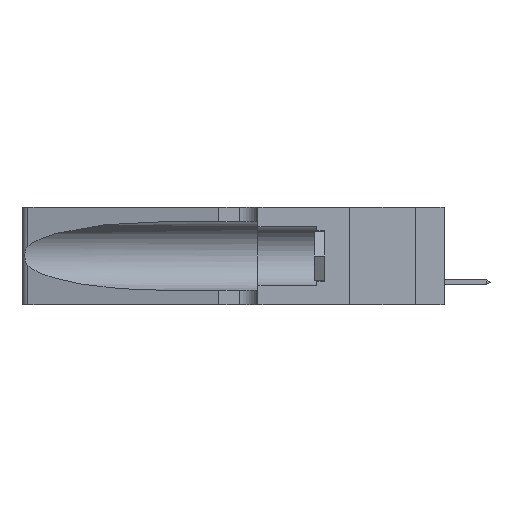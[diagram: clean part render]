
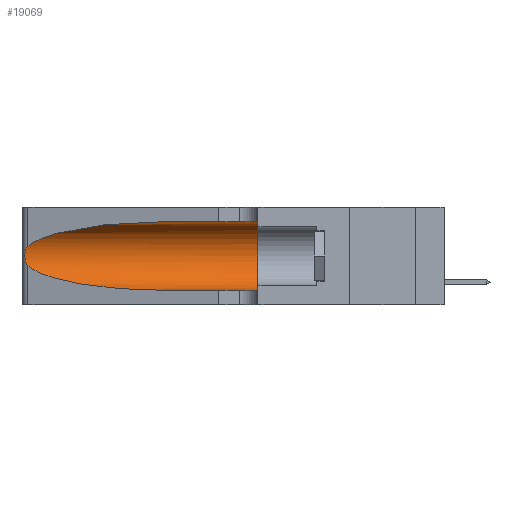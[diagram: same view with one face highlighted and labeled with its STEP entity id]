
A CAD part, left-side view. The second image highlights one B-rep face of the part: STEP entity #19069.
In plain terms, the highlighted cylindrical face has radius 3.308 mm (diameter 6.617 mm), a partial arc.
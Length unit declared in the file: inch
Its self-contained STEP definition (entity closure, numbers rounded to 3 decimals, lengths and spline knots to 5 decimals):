
#57 = CYLINDRICAL_SURFACE ( 'NONE', #22154, 0.13025 ) ;
#59 = CARTESIAN_POINT ( 'NONE',  ( 0.25639, 1.23184, 0.21858 ) ) ;
#171 = CARTESIAN_POINT ( 'NONE',  ( 0.18966, 0.96281, 0.05475 ) ) ;
#181 = CARTESIAN_POINT ( 'NONE',  ( 0.1305, 0.35, 0.31525 ) ) ;
#668 = DIRECTION ( 'NONE',  ( 0., -1., 0. ) ) ;
#1163 = VERTEX_POINT ( 'NONE', #20608 ) ;
#1965 = CARTESIAN_POINT ( 'NONE',  ( 0.1305, 1.61858, 0.05475 ) ) ;
#2052 = CARTESIAN_POINT ( 'NONE',  ( 0.1305, 0.35, 0.05475 ) ) ;
#2307 = CARTESIAN_POINT ( 'NONE',  ( 0.25639, 1.23186, 0.15144 ) ) ;
#3099 = VECTOR ( 'NONE', #668, 39.37008 ) ;
#3864 = EDGE_LOOP ( 'NONE', ( #15923, #24804, #15030, #12598, #13531, #11476 ) ) ;
#4411 = CARTESIAN_POINT ( 'NONE',  ( 0.25487, 1.22718, 0.14631 ) ) ;
#5501 = B_SPLINE_CURVE_WITH_KNOTS ( 'NONE', 3,
 ( #21310, #14853, #59, #8733, #10868, #6243, #8461, #10586, #12723, #23414, #21129, #2307, #16975, #4411 ),
 .UNSPECIFIED., .F., .F.,
 ( 4, 2, 2, 2, 2, 2, 4 ),
 ( 0., 0.00027, 0.00053, 0.00107, 0.0016, 0.00187, 0.00214 ),
 .UNSPECIFIED. ) ;
#6243 = CARTESIAN_POINT ( 'NONE',  ( 0.26018, 1.23835, 0.19895 ) ) ;
#6531 = CARTESIAN_POINT ( 'NONE',  ( 0.1305, 0.72297, 0.05475 ) ) ;
#7125 = CARTESIAN_POINT ( 'NONE',  ( 0.25487, 1.22718, 0.14631 ) ) ;
#7676 = FACE_OUTER_BOUND ( 'NONE', #3864, .T. ) ;
#7796 = CARTESIAN_POINT ( 'NONE',  ( 0.18966, 0.96281, 0.31525 ) ) ;
#8120 = DIRECTION ( 'NONE',  ( 0., -1., 0. ) ) ;
#8461 = CARTESIAN_POINT ( 'NONE',  ( 0.26075, 1.23896, 0.19203 ) ) ;
#8733 = CARTESIAN_POINT ( 'NONE',  ( 0.25787, 1.23484, 0.2124 ) ) ;
#10179 = DIRECTION ( 'NONE',  ( 0., 1., 0. ) ) ;
#10402 = CARTESIAN_POINT ( 'NONE',  ( 0.1305, 1.61858, 0.185 ) ) ;
#10586 = CARTESIAN_POINT ( 'NONE',  ( 0.26075, 1.23896, 0.178 ) ) ;
#10868 = CARTESIAN_POINT ( 'NONE',  ( 0.25854, 1.2359, 0.20912 ) ) ;
#11476 = ORIENTED_EDGE ( 'NONE', *, *, #18716, .F. ) ;
#12152 = CARTESIAN_POINT ( 'NONE',  ( 0.2373, 1.15595, 0.28018 ) ) ;
#12598 = ORIENTED_EDGE ( 'NONE', *, *, #16699, .T. ) ;
#12632 = AXIS2_PLACEMENT_3D ( 'NONE', #26853, #10179, #16386 ) ;
#12723 = CARTESIAN_POINT ( 'NONE',  ( 0.26017, 1.23833, 0.17102 ) ) ;
#13531 = ORIENTED_EDGE ( 'NONE', *, *, #16423, .F. ) ;
#14480 = CARTESIAN_POINT ( 'NONE',  ( 0.1305, 0.72297, 0.31525 ) ) ;
#14853 = CARTESIAN_POINT ( 'NONE',  ( 0.25555, 1.22994, 0.2215 ) ) ;
#15030 = ORIENTED_EDGE ( 'NONE', *, *, #16299, .T. ) ;
#15923 = ORIENTED_EDGE ( 'NONE', *, *, #20365, .T. ) ;
#16299 = EDGE_CURVE ( 'NONE', #19392, #17035, #22556, .T. ) ;
#16386 = DIRECTION ( 'NONE',  ( 0., 0., 1. ) ) ;
#16423 = EDGE_CURVE ( 'NONE', #18141, #23854, #26258, .T. ) ;
#16695 = DIRECTION ( 'NONE',  ( 0., 0., -1. ) ) ;
#16699 = EDGE_CURVE ( 'NONE', #17035, #23854, #21016, .T. ) ;
#16975 = CARTESIAN_POINT ( 'NONE',  ( 0.25555, 1.22993, 0.14849 ) ) ;
#17035 = VERTEX_POINT ( 'NONE', #23712 ) ;
#17803 = CARTESIAN_POINT ( 'NONE',  ( 0.25487, 1.22718, 0.14631 ) ) ;
#18141 = VERTEX_POINT ( 'NONE', #181 ) ;
#18259 = CARTESIAN_POINT ( 'NONE',  ( 0.25487, 1.22718, 0.22369 ) ) ;
#18561 = CARTESIAN_POINT ( 'NONE',  ( 0.25487, 1.22718, 0.22369 ) ) ;
#18716 = EDGE_CURVE ( 'NONE', #1163, #18141, #23797, .T. ) ;
#19069 = ADVANCED_FACE ( 'NONE', ( #7676 ), #57, .F. ) ;
#19392 = VERTEX_POINT ( 'NONE', #17803 ) ;
#19486 = CARTESIAN_POINT ( 'NONE',  ( 0.1305, 1.61858, 0.31525 ) ) ;
#20009 = VECTOR ( 'NONE', #8120, 39.37008 ) ;
#20365 = EDGE_CURVE ( 'NONE', #1163, #26180, #23028, .T. ) ;
#20608 = CARTESIAN_POINT ( 'NONE',  ( 0.1305, 0.72297, 0.31525 ) ) ;
#20979 = CARTESIAN_POINT ( 'NONE',  ( 0.2373, 1.15595, 0.08982 ) ) ;
#21016 = LINE ( 'NONE', #1965, #20009 ) ;
#21129 = CARTESIAN_POINT ( 'NONE',  ( 0.25789, 1.23486, 0.15765 ) ) ;
#21310 = CARTESIAN_POINT ( 'NONE',  ( 0.25487, 1.22718, 0.22369 ) ) ;
#22154 = AXIS2_PLACEMENT_3D ( 'NONE', #10402, #27161, #16695 ) ;
#22556 =( BOUNDED_CURVE ( )  B_SPLINE_CURVE ( 3, ( #7125, #20979, #171, #6531 ),
 .UNSPECIFIED., .F., .F. ) 
 B_SPLINE_CURVE_WITH_KNOTS ( ( 4, 4 ),
 ( 3.44316, 4.71239 ),
 .UNSPECIFIED. ) 
 CURVE ( )  GEOMETRIC_REPRESENTATION_ITEM ( )  RATIONAL_B_SPLINE_CURVE ( ( 1., 0.87, 0.87, 1. ) ) 
 REPRESENTATION_ITEM ( '' )  );
#23028 =( BOUNDED_CURVE ( )  B_SPLINE_CURVE ( 3, ( #14480, #7796, #12152, #18259 ),
 .UNSPECIFIED., .F., .F. ) 
 B_SPLINE_CURVE_WITH_KNOTS ( ( 4, 4 ),
 ( 1.5708, 2.84003 ),
 .UNSPECIFIED. ) 
 CURVE ( )  GEOMETRIC_REPRESENTATION_ITEM ( )  RATIONAL_B_SPLINE_CURVE ( ( 1., 0.87, 0.87, 1. ) ) 
 REPRESENTATION_ITEM ( '' )  );
#23414 = CARTESIAN_POINT ( 'NONE',  ( 0.25856, 1.23593, 0.16098 ) ) ;
#23712 = CARTESIAN_POINT ( 'NONE',  ( 0.1305, 0.72297, 0.05475 ) ) ;
#23797 = LINE ( 'NONE', #19486, #3099 ) ;
#23854 = VERTEX_POINT ( 'NONE', #2052 ) ;
#24804 = ORIENTED_EDGE ( 'NONE', *, *, #26364, .T. ) ;
#26180 = VERTEX_POINT ( 'NONE', #18561 ) ;
#26258 = CIRCLE ( 'NONE', #12632, 0.13025 ) ;
#26364 = EDGE_CURVE ( 'NONE', #26180, #19392, #5501, .T. ) ;
#26853 = CARTESIAN_POINT ( 'NONE',  ( 0.1305, 0.35, 0.185 ) ) ;
#27161 = DIRECTION ( 'NONE',  ( 0., -1., 0. ) ) ;
